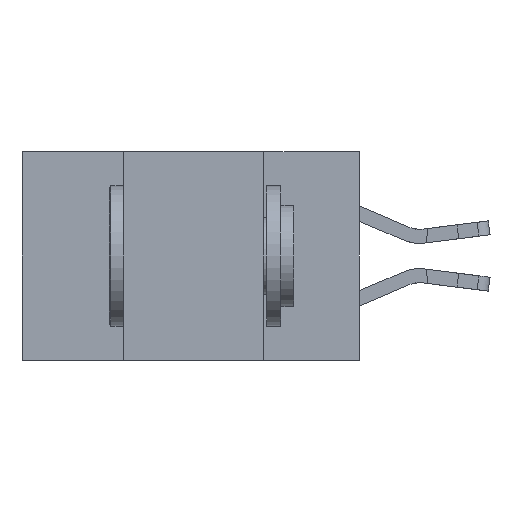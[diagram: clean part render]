
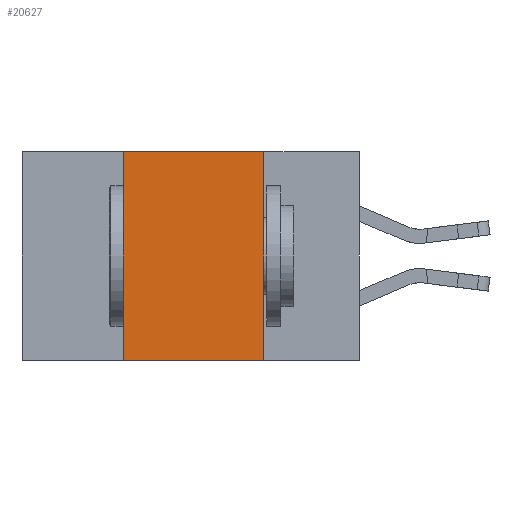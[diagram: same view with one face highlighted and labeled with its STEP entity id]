
A CAD part, left-side view. The second image highlights one B-rep face of the part: STEP entity #20627.
In plain terms, the highlighted planar face has unit normal (-1, 0, 0).
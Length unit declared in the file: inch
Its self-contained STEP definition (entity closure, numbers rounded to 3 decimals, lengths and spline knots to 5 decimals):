
#68 = PLANE ( 'NONE',  #24691 ) ;
#2133 = LINE ( 'NONE', #12788, #22042 ) ;
#3080 = EDGE_CURVE ( 'NONE', #20118, #24044, #2133, .T. ) ;
#4565 = EDGE_CURVE ( 'NONE', #20662, #18243, #6697, .T. ) ;
#5662 = VECTOR ( 'NONE', #12877, 39.37008 ) ;
#6078 = DIRECTION ( 'NONE',  ( 0., 0., -1. ) ) ;
#6552 = EDGE_LOOP ( 'NONE', ( #7211, #17963, #18547, #23635 ) ) ;
#6697 = LINE ( 'NONE', #10474, #11221 ) ;
#7211 = ORIENTED_EDGE ( 'NONE', *, *, #17700, .F. ) ;
#9041 = CARTESIAN_POINT ( 'NONE',  ( 0., 0.42, 0. ) ) ;
#9327 = DIRECTION ( 'NONE',  ( 0., 0., -1. ) ) ;
#10474 = CARTESIAN_POINT ( 'NONE',  ( 0., 0.6, -0.37 ) ) ;
#10755 = EDGE_CURVE ( 'NONE', #20662, #20118, #20332, .T. ) ;
#11221 = VECTOR ( 'NONE', #21976, 39.37008 ) ;
#12487 = CARTESIAN_POINT ( 'NONE',  ( 0., 0.17, 0. ) ) ;
#12788 = CARTESIAN_POINT ( 'NONE',  ( 0., 0.6, 0. ) ) ;
#12877 = DIRECTION ( 'NONE',  ( 0., 0., 1. ) ) ;
#13974 = LINE ( 'NONE', #22664, #18413 ) ;
#16947 = CARTESIAN_POINT ( 'NONE',  ( 0., 0.17, -0.37 ) ) ;
#17531 = DIRECTION ( 'NONE',  ( 1., 0., 0. ) ) ;
#17700 = EDGE_CURVE ( 'NONE', #24044, #18243, #13974, .T. ) ;
#17963 = ORIENTED_EDGE ( 'NONE', *, *, #3080, .F. ) ;
#18208 = DIRECTION ( 'NONE',  ( 0., -1., 0. ) ) ;
#18243 = VERTEX_POINT ( 'NONE', #16947 ) ;
#18413 = VECTOR ( 'NONE', #9327, 39.37008 ) ;
#18547 = ORIENTED_EDGE ( 'NONE', *, *, #10755, .F. ) ;
#19455 = CARTESIAN_POINT ( 'NONE',  ( 0., 0.42, -0.37 ) ) ;
#20118 = VERTEX_POINT ( 'NONE', #21761 ) ;
#20332 = LINE ( 'NONE', #9041, #5662 ) ;
#20627 = ADVANCED_FACE ( 'NONE', ( #22477 ), #68, .F. ) ;
#20662 = VERTEX_POINT ( 'NONE', #19455 ) ;
#21312 = CARTESIAN_POINT ( 'NONE',  ( 0., 0.6, 0. ) ) ;
#21761 = CARTESIAN_POINT ( 'NONE',  ( 0., 0.42, 0. ) ) ;
#21976 = DIRECTION ( 'NONE',  ( 0., -1., 0. ) ) ;
#22042 = VECTOR ( 'NONE', #18208, 39.37008 ) ;
#22477 = FACE_OUTER_BOUND ( 'NONE', #6552, .T. ) ;
#22664 = CARTESIAN_POINT ( 'NONE',  ( 0., 0.17, 0. ) ) ;
#23635 = ORIENTED_EDGE ( 'NONE', *, *, #4565, .T. ) ;
#24044 = VERTEX_POINT ( 'NONE', #12487 ) ;
#24691 = AXIS2_PLACEMENT_3D ( 'NONE', #21312, #17531, #6078 ) ;
